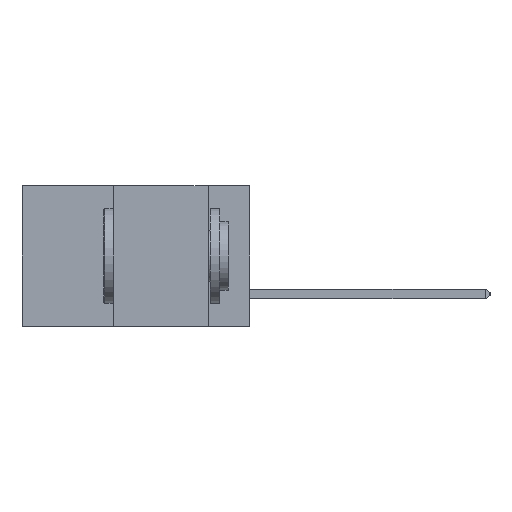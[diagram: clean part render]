
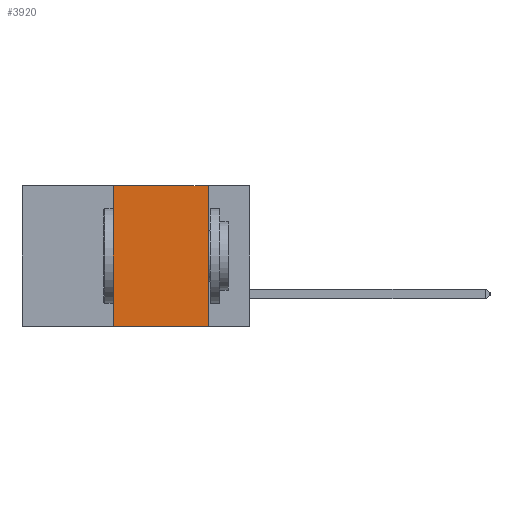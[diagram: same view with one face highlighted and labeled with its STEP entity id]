
A CAD part, left-side view. The second image highlights one B-rep face of the part: STEP entity #3920.
In plain terms, the highlighted planar face has unit normal (-1, 0, 0).
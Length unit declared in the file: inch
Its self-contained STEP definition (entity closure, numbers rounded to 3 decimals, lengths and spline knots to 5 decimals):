
#613 = VERTEX_POINT ( 'NONE', #5109 ) ;
#743 = EDGE_CURVE ( 'NONE', #17036, #5668, #5294, .T. ) ;
#810 = AXIS2_PLACEMENT_3D ( 'NONE', #9066, #9029, #9026 ) ;
#842 = EDGE_LOOP ( 'NONE', ( #16837, #13671, #12928, #8995 ) ) ;
#1653 = VECTOR ( 'NONE', #15497, 39.37008 ) ;
#1875 = CARTESIAN_POINT ( 'NONE',  ( 0., 0.6, 0. ) ) ;
#1959 = CARTESIAN_POINT ( 'NONE',  ( 0., 0.36, 0. ) ) ;
#2046 = LINE ( 'NONE', #12050, #4825 ) ;
#3683 = CARTESIAN_POINT ( 'NONE',  ( 0., 0.36, -0.37 ) ) ;
#3915 = FACE_OUTER_BOUND ( 'NONE', #842, .T. ) ;
#3920 = ADVANCED_FACE ( 'NONE', ( #3915 ), #9199, .F. ) ;
#3931 = VERTEX_POINT ( 'NONE', #8920 ) ;
#4825 = VECTOR ( 'NONE', #13394, 39.37008 ) ;
#5109 = CARTESIAN_POINT ( 'NONE',  ( 0., 0.11, -0.37 ) ) ;
#5188 = CARTESIAN_POINT ( 'NONE',  ( 0., 0.36, 0. ) ) ;
#5294 = LINE ( 'NONE', #1959, #11237 ) ;
#5668 = VERTEX_POINT ( 'NONE', #5188 ) ;
#8920 = CARTESIAN_POINT ( 'NONE',  ( 0., 0.11, 0. ) ) ;
#8995 = ORIENTED_EDGE ( 'NONE', *, *, #16881, .T. ) ;
#9026 = DIRECTION ( 'NONE',  ( 0., 0., -1. ) ) ;
#9029 = DIRECTION ( 'NONE',  ( 1., 0., 0. ) ) ;
#9066 = CARTESIAN_POINT ( 'NONE',  ( 0., 0.6, 0. ) ) ;
#9199 = PLANE ( 'NONE',  #810 ) ;
#9303 = LINE ( 'NONE', #14155, #1653 ) ;
#10074 = DIRECTION ( 'NONE',  ( 0., -1., 0. ) ) ;
#11237 = VECTOR ( 'NONE', #11801, 39.37008 ) ;
#11800 = EDGE_CURVE ( 'NONE', #3931, #613, #2046, .T. ) ;
#11801 = DIRECTION ( 'NONE',  ( 0., 0., 1. ) ) ;
#12050 = CARTESIAN_POINT ( 'NONE',  ( 0., 0.11, 0. ) ) ;
#12928 = ORIENTED_EDGE ( 'NONE', *, *, #743, .F. ) ;
#13394 = DIRECTION ( 'NONE',  ( 0., 0., -1. ) ) ;
#13671 = ORIENTED_EDGE ( 'NONE', *, *, #13894, .F. ) ;
#13873 = VECTOR ( 'NONE', #10074, 39.37008 ) ;
#13894 = EDGE_CURVE ( 'NONE', #5668, #3931, #17424, .T. ) ;
#14155 = CARTESIAN_POINT ( 'NONE',  ( 0., 0.6, -0.37 ) ) ;
#15497 = DIRECTION ( 'NONE',  ( 0., -1., 0. ) ) ;
#16837 = ORIENTED_EDGE ( 'NONE', *, *, #11800, .F. ) ;
#16881 = EDGE_CURVE ( 'NONE', #17036, #613, #9303, .T. ) ;
#17036 = VERTEX_POINT ( 'NONE', #3683 ) ;
#17424 = LINE ( 'NONE', #1875, #13873 ) ;
